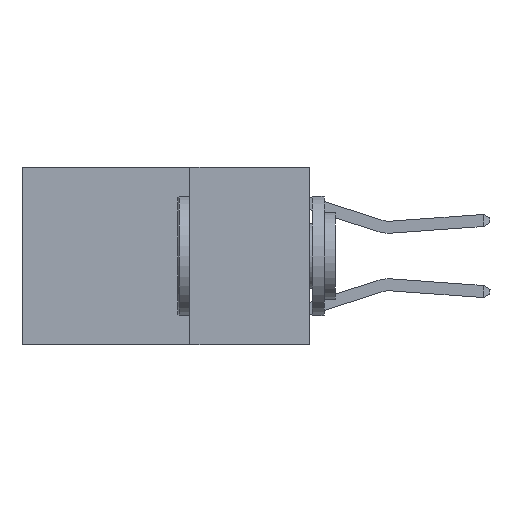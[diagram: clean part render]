
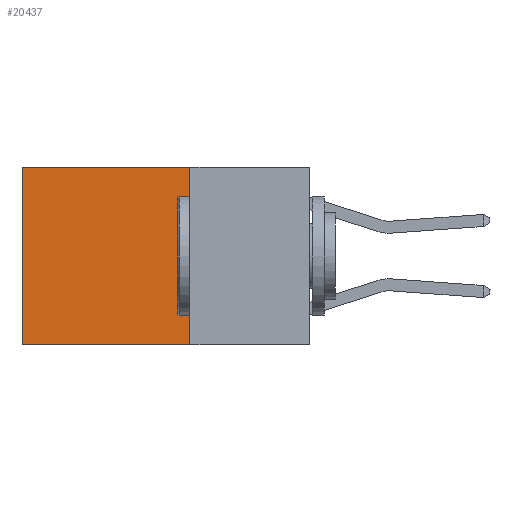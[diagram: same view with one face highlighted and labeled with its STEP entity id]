
A CAD part, left-side view. The second image highlights one B-rep face of the part: STEP entity #20437.
In plain terms, the highlighted planar face has unit normal (-1, 0, 0).
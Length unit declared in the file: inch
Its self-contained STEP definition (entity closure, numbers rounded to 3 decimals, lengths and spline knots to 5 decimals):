
#57 = CARTESIAN_POINT ( 'NONE',  ( 0.2625, 0.6, 0. ) ) ;
#528 = CARTESIAN_POINT ( 'NONE',  ( 0.2625, 0.25, 0. ) ) ;
#1284 = VERTEX_POINT ( 'NONE', #19094 ) ;
#2344 = ORIENTED_EDGE ( 'NONE', *, *, #26716, .F. ) ;
#2718 = VECTOR ( 'NONE', #20367, 39.37008 ) ;
#2778 = EDGE_CURVE ( 'NONE', #6914, #20950, #15397, .T. ) ;
#2905 = PLANE ( 'NONE',  #26300 ) ;
#3696 = VECTOR ( 'NONE', #6362, 39.37008 ) ;
#4293 = LINE ( 'NONE', #8292, #26045 ) ;
#5077 = DIRECTION ( 'NONE',  ( 0., 0., -1. ) ) ;
#6362 = DIRECTION ( 'NONE',  ( 0., 1., 0. ) ) ;
#6806 = ORIENTED_EDGE ( 'NONE', *, *, #18074, .F. ) ;
#6914 = VERTEX_POINT ( 'NONE', #528 ) ;
#8292 = CARTESIAN_POINT ( 'NONE',  ( 0.2625, 0.25, -0.37 ) ) ;
#8732 = CARTESIAN_POINT ( 'NONE',  ( 0.2625, 0.6, -0.37 ) ) ;
#9304 = EDGE_LOOP ( 'NONE', ( #10205, #6806, #2344, #19979 ) ) ;
#9604 = LINE ( 'NONE', #15812, #26142 ) ;
#10205 = ORIENTED_EDGE ( 'NONE', *, *, #16236, .T. ) ;
#10239 = VERTEX_POINT ( 'NONE', #8732 ) ;
#15093 = LINE ( 'NONE', #26799, #2718 ) ;
#15397 = LINE ( 'NONE', #21604, #3696 ) ;
#15812 = CARTESIAN_POINT ( 'NONE',  ( 0.2625, 0.25, 0. ) ) ;
#16236 = EDGE_CURVE ( 'NONE', #20950, #10239, #15093, .T. ) ;
#18074 = EDGE_CURVE ( 'NONE', #1284, #10239, #4293, .T. ) ;
#18209 = DIRECTION ( 'NONE',  ( 1., 0., 0. ) ) ;
#19094 = CARTESIAN_POINT ( 'NONE',  ( 0.2625, 0.25, -0.37 ) ) ;
#19614 = FACE_OUTER_BOUND ( 'NONE', #9304, .T. ) ;
#19979 = ORIENTED_EDGE ( 'NONE', *, *, #2778, .T. ) ;
#20367 = DIRECTION ( 'NONE',  ( 0., 0., -1. ) ) ;
#20437 = ADVANCED_FACE ( 'NONE', ( #19614 ), #2905, .F. ) ;
#20950 = VERTEX_POINT ( 'NONE', #57 ) ;
#21604 = CARTESIAN_POINT ( 'NONE',  ( 0.2625, 0.25, 0. ) ) ;
#22324 = DIRECTION ( 'NONE',  ( 0., 0., -1. ) ) ;
#24575 = CARTESIAN_POINT ( 'NONE',  ( 0.2625, 0.25, 0. ) ) ;
#25594 = DIRECTION ( 'NONE',  ( 0., 1., 0. ) ) ;
#26045 = VECTOR ( 'NONE', #25594, 39.37008 ) ;
#26142 = VECTOR ( 'NONE', #22324, 39.37008 ) ;
#26300 = AXIS2_PLACEMENT_3D ( 'NONE', #24575, #18209, #5077 ) ;
#26716 = EDGE_CURVE ( 'NONE', #6914, #1284, #9604, .T. ) ;
#26799 = CARTESIAN_POINT ( 'NONE',  ( 0.2625, 0.6, 0. ) ) ;
